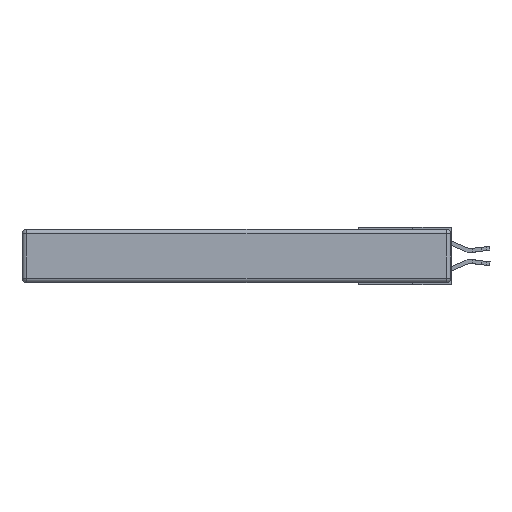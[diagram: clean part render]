
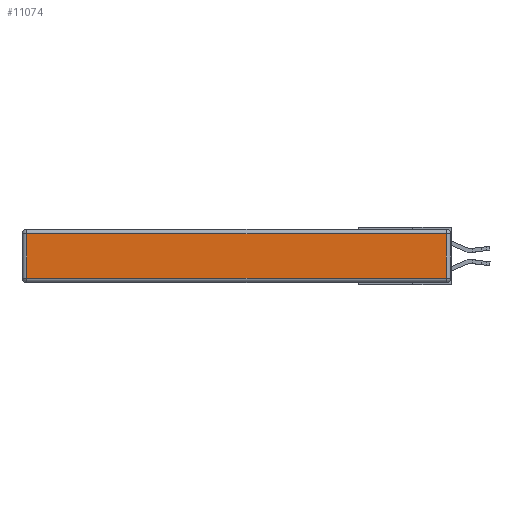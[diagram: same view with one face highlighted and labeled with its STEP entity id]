
A CAD part, left-side view. The second image highlights one B-rep face of the part: STEP entity #11074.
In plain terms, the highlighted planar face has unit normal (-1, 0, 0).
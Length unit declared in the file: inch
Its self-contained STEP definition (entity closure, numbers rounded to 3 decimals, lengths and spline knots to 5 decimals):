
#1068 = DIRECTION ( 'NONE',  ( 0., 0., -1. ) ) ;
#1839 = DIRECTION ( 'NONE',  ( -1., 0., 0. ) ) ;
#2870 = CARTESIAN_POINT ( 'NONE',  ( 0., 0.03, -0.343 ) ) ;
#3092 = EDGE_CURVE ( 'NONE', #12717, #16704, #15985, .T. ) ;
#4220 = ORIENTED_EDGE ( 'NONE', *, *, #8175, .T. ) ;
#5548 = DIRECTION ( 'NONE',  ( 0., -1., 0. ) ) ;
#5549 = CARTESIAN_POINT ( 'NONE',  ( 0., 0.03, -0.03 ) ) ;
#5852 = CARTESIAN_POINT ( 'NONE',  ( 0., 0., -0.343 ) ) ;
#6817 = CARTESIAN_POINT ( 'NONE',  ( 0., 2.72, -0.343 ) ) ;
#7707 = ORIENTED_EDGE ( 'NONE', *, *, #19444, .T. ) ;
#8133 = LINE ( 'NONE', #2870, #24185 ) ;
#8175 = EDGE_CURVE ( 'NONE', #22884, #12717, #17114, .T. ) ;
#9311 = EDGE_LOOP ( 'NONE', ( #7707, #11706, #4220, #19437 ) ) ;
#9367 = CARTESIAN_POINT ( 'NONE',  ( 0., 2.72, -0.313 ) ) ;
#9382 = PLANE ( 'NONE',  #23554 ) ;
#10597 = VECTOR ( 'NONE', #1068, 39.37008 ) ;
#11074 = ADVANCED_FACE ( 'NONE', ( #22022 ), #9382, .T. ) ;
#11706 = ORIENTED_EDGE ( 'NONE', *, *, #13081, .T. ) ;
#12558 = DIRECTION ( 'NONE',  ( 0., 0., 1. ) ) ;
#12717 = VERTEX_POINT ( 'NONE', #16797 ) ;
#12886 = DIRECTION ( 'NONE',  ( 0., 1., 0. ) ) ;
#12925 = LINE ( 'NONE', #16884, #14447 ) ;
#12998 = CARTESIAN_POINT ( 'NONE',  ( 0., 0.03, -0.313 ) ) ;
#13081 = EDGE_CURVE ( 'NONE', #16755, #22884, #8133, .T. ) ;
#13552 = VECTOR ( 'NONE', #12886, 39.37008 ) ;
#14447 = VECTOR ( 'NONE', #5548, 39.37008 ) ;
#15985 = LINE ( 'NONE', #6817, #10597 ) ;
#16704 = VERTEX_POINT ( 'NONE', #9367 ) ;
#16755 = VERTEX_POINT ( 'NONE', #12998 ) ;
#16797 = CARTESIAN_POINT ( 'NONE',  ( 0., 2.72, -0.03 ) ) ;
#16884 = CARTESIAN_POINT ( 'NONE',  ( 0., 0., -0.313 ) ) ;
#17114 = LINE ( 'NONE', #24178, #13552 ) ;
#19437 = ORIENTED_EDGE ( 'NONE', *, *, #3092, .T. ) ;
#19444 = EDGE_CURVE ( 'NONE', #16704, #16755, #12925, .T. ) ;
#22022 = FACE_OUTER_BOUND ( 'NONE', #9311, .T. ) ;
#22884 = VERTEX_POINT ( 'NONE', #5549 ) ;
#23554 = AXIS2_PLACEMENT_3D ( 'NONE', #5852, #1839, #24662 ) ;
#24178 = CARTESIAN_POINT ( 'NONE',  ( 0., 2.75, -0.03 ) ) ;
#24185 = VECTOR ( 'NONE', #12558, 39.37008 ) ;
#24662 = DIRECTION ( 'NONE',  ( 0., 0., 1. ) ) ;
